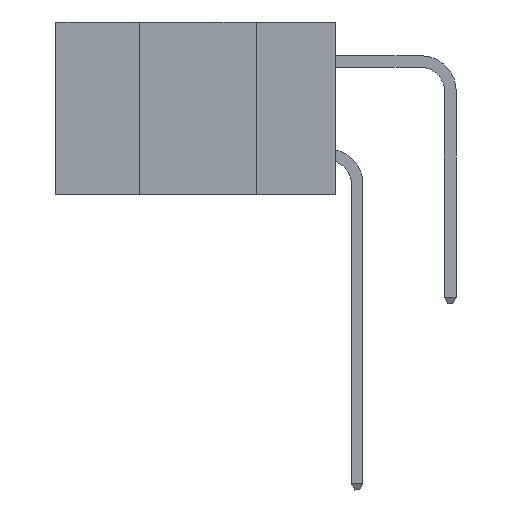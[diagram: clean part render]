
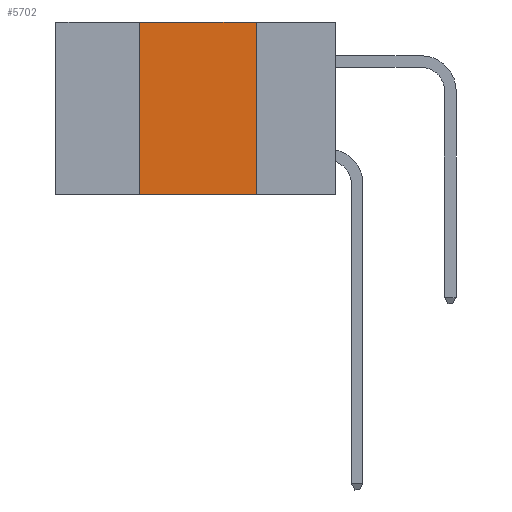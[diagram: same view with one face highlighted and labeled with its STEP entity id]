
A CAD part, left-side view. The second image highlights one B-rep face of the part: STEP entity #5702.
In plain terms, the highlighted planar face has unit normal (-1, 0, 0).
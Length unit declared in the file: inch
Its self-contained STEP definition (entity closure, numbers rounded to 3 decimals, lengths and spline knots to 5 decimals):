
#523 = CARTESIAN_POINT ( 'NONE',  ( 0., 0.42, 0. ) ) ;
#792 = EDGE_CURVE ( 'NONE', #8289, #12055, #18588, .T. ) ;
#862 = LINE ( 'NONE', #18109, #19819 ) ;
#1401 = CARTESIAN_POINT ( 'NONE',  ( 0., 0.17, 0. ) ) ;
#1557 = VECTOR ( 'NONE', #4552, 39.37008 ) ;
#3369 = ORIENTED_EDGE ( 'NONE', *, *, #4989, .F. ) ;
#4087 = DIRECTION ( 'NONE',  ( 0., 0., -1. ) ) ;
#4175 = DIRECTION ( 'NONE',  ( 0., -1., 0. ) ) ;
#4252 = AXIS2_PLACEMENT_3D ( 'NONE', #7208, #12498, #4087 ) ;
#4420 = CARTESIAN_POINT ( 'NONE',  ( 0., 0.6, -0.37 ) ) ;
#4552 = DIRECTION ( 'NONE',  ( 0., 0., -1. ) ) ;
#4989 = EDGE_CURVE ( 'NONE', #8289, #8761, #6541, .T. ) ;
#5688 = VERTEX_POINT ( 'NONE', #1401 ) ;
#5702 = ADVANCED_FACE ( 'NONE', ( #14301 ), #21255, .F. ) ;
#5803 = EDGE_LOOP ( 'NONE', ( #7781, #9210, #3369, #17882 ) ) ;
#6541 = LINE ( 'NONE', #20742, #11096 ) ;
#6803 = CARTESIAN_POINT ( 'NONE',  ( 0., 0.17, -0.37 ) ) ;
#7208 = CARTESIAN_POINT ( 'NONE',  ( 0., 0.6, 0. ) ) ;
#7781 = ORIENTED_EDGE ( 'NONE', *, *, #20895, .F. ) ;
#8289 = VERTEX_POINT ( 'NONE', #16667 ) ;
#8572 = DIRECTION ( 'NONE',  ( 0., 0., 1. ) ) ;
#8761 = VERTEX_POINT ( 'NONE', #523 ) ;
#9175 = EDGE_CURVE ( 'NONE', #8761, #5688, #862, .T. ) ;
#9210 = ORIENTED_EDGE ( 'NONE', *, *, #9175, .F. ) ;
#11037 = LINE ( 'NONE', #14916, #1557 ) ;
#11096 = VECTOR ( 'NONE', #8572, 39.37008 ) ;
#12055 = VERTEX_POINT ( 'NONE', #6803 ) ;
#12498 = DIRECTION ( 'NONE',  ( 1., 0., 0. ) ) ;
#14301 = FACE_OUTER_BOUND ( 'NONE', #5803, .T. ) ;
#14916 = CARTESIAN_POINT ( 'NONE',  ( 0., 0.17, 0. ) ) ;
#16667 = CARTESIAN_POINT ( 'NONE',  ( 0., 0.42, -0.37 ) ) ;
#17882 = ORIENTED_EDGE ( 'NONE', *, *, #792, .T. ) ;
#18109 = CARTESIAN_POINT ( 'NONE',  ( 0., 0.6, 0. ) ) ;
#18244 = DIRECTION ( 'NONE',  ( 0., -1., 0. ) ) ;
#18588 = LINE ( 'NONE', #4420, #19138 ) ;
#19138 = VECTOR ( 'NONE', #18244, 39.37008 ) ;
#19819 = VECTOR ( 'NONE', #4175, 39.37008 ) ;
#20742 = CARTESIAN_POINT ( 'NONE',  ( 0., 0.42, 0. ) ) ;
#20895 = EDGE_CURVE ( 'NONE', #5688, #12055, #11037, .T. ) ;
#21255 = PLANE ( 'NONE',  #4252 ) ;
